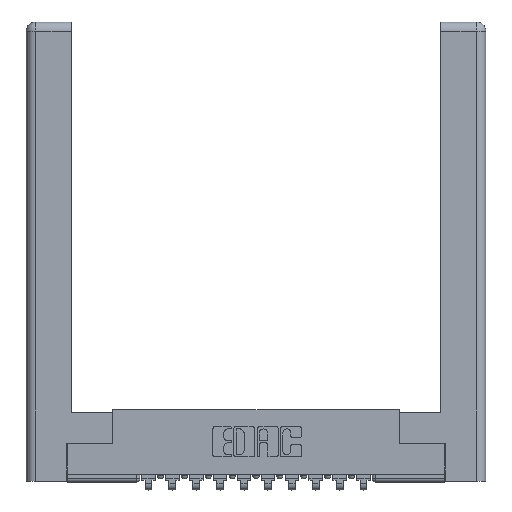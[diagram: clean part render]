
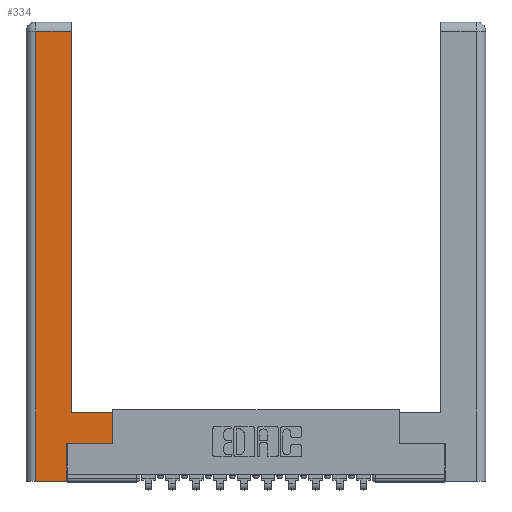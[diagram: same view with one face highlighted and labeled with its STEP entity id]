
A CAD part, top view. The second image highlights one B-rep face of the part: STEP entity #334.
In plain terms, the highlighted planar face has unit normal (0, 0, 1).
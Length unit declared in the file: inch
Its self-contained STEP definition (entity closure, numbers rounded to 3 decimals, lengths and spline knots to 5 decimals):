
#45 = EDGE_CURVE ( 'NONE', #12767, #2755, #9279, .T. ) ;
#241 = DIRECTION ( 'NONE',  ( 1., 0., 0. ) ) ;
#278 = DIRECTION ( 'NONE',  ( -1., 0., 0. ) ) ;
#334 = ADVANCED_FACE ( 'NONE', ( #5002 ), #6296, .F. ) ;
#343 = EDGE_CURVE ( 'NONE', #7893, #5599, #3787, .T. ) ;
#1422 = LINE ( 'NONE', #11354, #2566 ) ;
#1508 = CARTESIAN_POINT ( 'NONE',  ( 0.265, 0.245, 0. ) ) ;
#1916 = DIRECTION ( 'NONE',  ( 0., 1., 0. ) ) ;
#1951 = ORIENTED_EDGE ( 'NONE', *, *, #7456, .T. ) ;
#2566 = VECTOR ( 'NONE', #278, 39.37008 ) ;
#2585 = VERTEX_POINT ( 'NONE', #5952 ) ;
#2622 = DIRECTION ( 'NONE',  ( 1., 0., 0. ) ) ;
#2632 = DIRECTION ( 'NONE',  ( 0., -1., 0. ) ) ;
#2755 = VERTEX_POINT ( 'NONE', #8755 ) ;
#3527 = EDGE_CURVE ( 'NONE', #7690, #12767, #1422, .T. ) ;
#3598 = AXIS2_PLACEMENT_3D ( 'NONE', #11360, #14868, #7508 ) ;
#3787 = LINE ( 'NONE', #1508, #13420 ) ;
#3843 = VECTOR ( 'NONE', #2632, 39.37008 ) ;
#3844 = LINE ( 'NONE', #10129, #15024 ) ;
#3949 = CARTESIAN_POINT ( 'NONE',  ( 0.0615, 2.94, 0. ) ) ;
#4336 = LINE ( 'NONE', #7892, #14530 ) ;
#4398 = EDGE_CURVE ( 'NONE', #13002, #7893, #13765, .T. ) ;
#4854 = EDGE_CURVE ( 'NONE', #14671, #7690, #4336, .T. ) ;
#5002 = FACE_OUTER_BOUND ( 'NONE', #6852, .T. ) ;
#5042 = CARTESIAN_POINT ( 'NONE',  ( 0.265, 0., 0. ) ) ;
#5164 = ORIENTED_EDGE ( 'NONE', *, *, #15165, .T. ) ;
#5316 = ORIENTED_EDGE ( 'NONE', *, *, #3527, .T. ) ;
#5599 = VERTEX_POINT ( 'NONE', #12741 ) ;
#5668 = ORIENTED_EDGE ( 'NONE', *, *, #343, .T. ) ;
#5952 = CARTESIAN_POINT ( 'NONE',  ( 0.0615, 2.94, 0. ) ) ;
#6296 = PLANE ( 'NONE',  #3598 ) ;
#6852 = EDGE_LOOP ( 'NONE', ( #9538, #5164, #10069, #8121, #5668, #1951, #12446, #5316 ) ) ;
#7456 = EDGE_CURVE ( 'NONE', #5599, #14671, #3844, .T. ) ;
#7508 = DIRECTION ( 'NONE',  ( -1., 0., 0. ) ) ;
#7587 = LINE ( 'NONE', #3949, #13122 ) ;
#7641 = CARTESIAN_POINT ( 'NONE',  ( 0.0615, 0., 0. ) ) ;
#7690 = VERTEX_POINT ( 'NONE', #9478 ) ;
#7892 = CARTESIAN_POINT ( 'NONE',  ( 0.565, 0.45, 0. ) ) ;
#7893 = VERTEX_POINT ( 'NONE', #5042 ) ;
#8121 = ORIENTED_EDGE ( 'NONE', *, *, #4398, .T. ) ;
#8649 = CARTESIAN_POINT ( 'NONE',  ( 0.565, 0.245, 0. ) ) ;
#8707 = DIRECTION ( 'NONE',  ( 0., 1., 0. ) ) ;
#8755 = CARTESIAN_POINT ( 'NONE',  ( 0.295, 2.94, 0. ) ) ;
#9279 = LINE ( 'NONE', #11785, #11193 ) ;
#9478 = CARTESIAN_POINT ( 'NONE',  ( 0.565, 0.45, 0. ) ) ;
#9538 = ORIENTED_EDGE ( 'NONE', *, *, #45, .T. ) ;
#10030 = CARTESIAN_POINT ( 'NONE',  ( 0.265, 0., 0. ) ) ;
#10069 = ORIENTED_EDGE ( 'NONE', *, *, #15592, .T. ) ;
#10129 = CARTESIAN_POINT ( 'NONE',  ( 0.565, 0.245, 0. ) ) ;
#10567 = VECTOR ( 'NONE', #241, 39.37008 ) ;
#10571 = CARTESIAN_POINT ( 'NONE',  ( 0.295, 0.45, 0. ) ) ;
#11193 = VECTOR ( 'NONE', #1916, 39.37008 ) ;
#11346 = LINE ( 'NONE', #7641, #3843 ) ;
#11354 = CARTESIAN_POINT ( 'NONE',  ( 0.295, 0.45, 0. ) ) ;
#11360 = CARTESIAN_POINT ( 'NONE',  ( 0., 0., 0. ) ) ;
#11785 = CARTESIAN_POINT ( 'NONE',  ( 0.295, 3., 0. ) ) ;
#12446 = ORIENTED_EDGE ( 'NONE', *, *, #4854, .T. ) ;
#12741 = CARTESIAN_POINT ( 'NONE',  ( 0.265, 0.245, 0. ) ) ;
#12767 = VERTEX_POINT ( 'NONE', #10571 ) ;
#12836 = DIRECTION ( 'NONE',  ( 0., 1., 0. ) ) ;
#13002 = VERTEX_POINT ( 'NONE', #15844 ) ;
#13122 = VECTOR ( 'NONE', #13891, 39.37008 ) ;
#13420 = VECTOR ( 'NONE', #8707, 39.37008 ) ;
#13765 = LINE ( 'NONE', #10030, #10567 ) ;
#13891 = DIRECTION ( 'NONE',  ( -1., 0., 0. ) ) ;
#14530 = VECTOR ( 'NONE', #12836, 39.37008 ) ;
#14671 = VERTEX_POINT ( 'NONE', #8649 ) ;
#14868 = DIRECTION ( 'NONE',  ( 0., 0., -1. ) ) ;
#15024 = VECTOR ( 'NONE', #2622, 39.37008 ) ;
#15165 = EDGE_CURVE ( 'NONE', #2755, #2585, #7587, .T. ) ;
#15592 = EDGE_CURVE ( 'NONE', #2585, #13002, #11346, .T. ) ;
#15844 = CARTESIAN_POINT ( 'NONE',  ( 0.0615, 0., 0. ) ) ;
